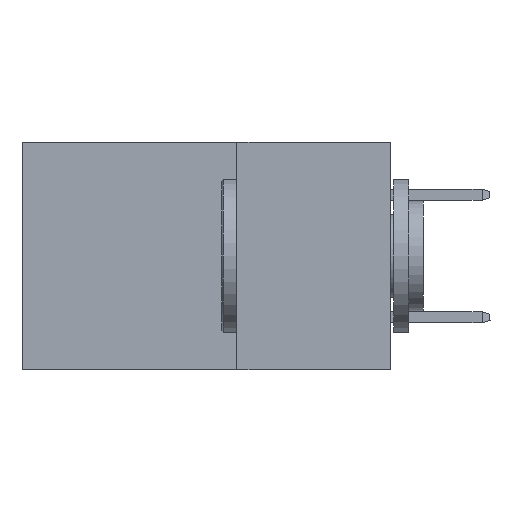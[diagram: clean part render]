
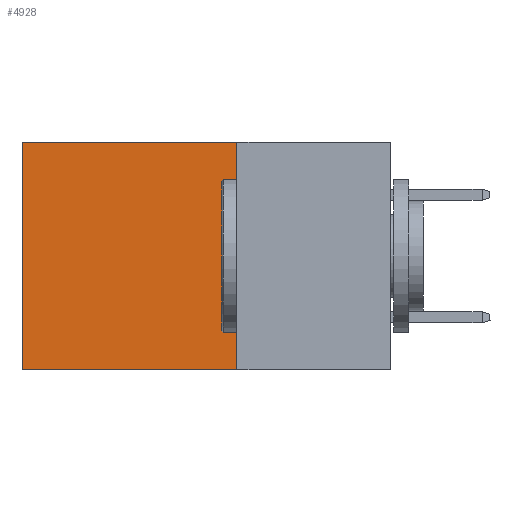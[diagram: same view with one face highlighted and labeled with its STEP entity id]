
A CAD part, left-side view. The second image highlights one B-rep face of the part: STEP entity #4928.
In plain terms, the highlighted planar face has unit normal (-1, 0, 0).
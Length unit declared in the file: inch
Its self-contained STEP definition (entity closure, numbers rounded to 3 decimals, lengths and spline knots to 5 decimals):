
#1117 = VERTEX_POINT ( 'NONE', #9521 ) ;
#1240 = EDGE_CURVE ( 'NONE', #6481, #3423, #16171, .T. ) ;
#1800 = AXIS2_PLACEMENT_3D ( 'NONE', #30778, #8976, #9337 ) ;
#3423 = VERTEX_POINT ( 'NONE', #4751 ) ;
#4751 = CARTESIAN_POINT ( 'NONE',  ( 0.2875, 0.6, -0.37 ) ) ;
#4928 = ADVANCED_FACE ( 'NONE', ( #6617 ), #21505, .F. ) ;
#6481 = VERTEX_POINT ( 'NONE', #16614 ) ;
#6617 = FACE_OUTER_BOUND ( 'NONE', #9808, .T. ) ;
#8019 = VECTOR ( 'NONE', #30204, 39.37008 ) ;
#8976 = DIRECTION ( 'NONE',  ( 1., 0., 0. ) ) ;
#9337 = DIRECTION ( 'NONE',  ( 0., 0., -1. ) ) ;
#9521 = CARTESIAN_POINT ( 'NONE',  ( 0.2875, 0.25, -0.37 ) ) ;
#9734 = ORIENTED_EDGE ( 'NONE', *, *, #20088, .T. ) ;
#9808 = EDGE_LOOP ( 'NONE', ( #30978, #16725, #11861, #9734 ) ) ;
#10373 = DIRECTION ( 'NONE',  ( 0., 0., -1. ) ) ;
#11530 = DIRECTION ( 'NONE',  ( 0., 1., 0. ) ) ;
#11861 = ORIENTED_EDGE ( 'NONE', *, *, #20414, .F. ) ;
#12486 = VERTEX_POINT ( 'NONE', #16534 ) ;
#12935 = EDGE_CURVE ( 'NONE', #1117, #3423, #20994, .T. ) ;
#13310 = LINE ( 'NONE', #26124, #22915 ) ;
#14055 = VECTOR ( 'NONE', #10373, 39.37008 ) ;
#15677 = DIRECTION ( 'NONE',  ( 0., 1., 0. ) ) ;
#16171 = LINE ( 'NONE', #29514, #8019 ) ;
#16534 = CARTESIAN_POINT ( 'NONE',  ( 0.2875, 0.25, 0. ) ) ;
#16614 = CARTESIAN_POINT ( 'NONE',  ( 0.2875, 0.6, 0. ) ) ;
#16725 = ORIENTED_EDGE ( 'NONE', *, *, #12935, .F. ) ;
#20088 = EDGE_CURVE ( 'NONE', #12486, #6481, #13310, .T. ) ;
#20197 = VECTOR ( 'NONE', #15677, 39.37008 ) ;
#20414 = EDGE_CURVE ( 'NONE', #12486, #1117, #30968, .T. ) ;
#20994 = LINE ( 'NONE', #30382, #20197 ) ;
#21505 = PLANE ( 'NONE',  #1800 ) ;
#22915 = VECTOR ( 'NONE', #11530, 39.37008 ) ;
#24964 = CARTESIAN_POINT ( 'NONE',  ( 0.2875, 0.25, 0. ) ) ;
#26124 = CARTESIAN_POINT ( 'NONE',  ( 0.2875, 0.25, 0. ) ) ;
#29514 = CARTESIAN_POINT ( 'NONE',  ( 0.2875, 0.6, 0. ) ) ;
#30204 = DIRECTION ( 'NONE',  ( 0., 0., -1. ) ) ;
#30382 = CARTESIAN_POINT ( 'NONE',  ( 0.2875, 0.25, -0.37 ) ) ;
#30778 = CARTESIAN_POINT ( 'NONE',  ( 0.2875, 0.25, 0. ) ) ;
#30968 = LINE ( 'NONE', #24964, #14055 ) ;
#30978 = ORIENTED_EDGE ( 'NONE', *, *, #1240, .T. ) ;
